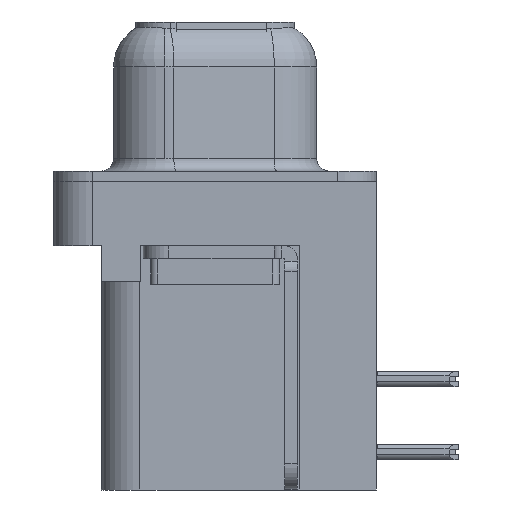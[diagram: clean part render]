
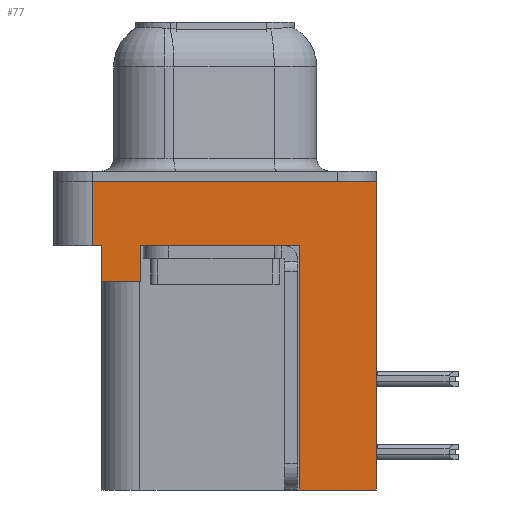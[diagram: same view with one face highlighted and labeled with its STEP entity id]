
A CAD part, left-side view. The second image highlights one B-rep face of the part: STEP entity #77.
In plain terms, the highlighted planar face has unit normal (-1, 0, 0).
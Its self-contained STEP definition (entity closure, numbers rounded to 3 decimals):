
#77 = ADVANCED_FACE ( 'NONE', ( #7146 ), #19064, .T. ) ;
#356 = LINE ( 'NONE', #5273, #6359 ) ;
#1047 = EDGE_CURVE ( 'NONE', #13381, #5297, #17923, .T. ) ;
#1210 = ORIENTED_EDGE ( 'NONE', *, *, #11453, .F. ) ;
#1944 = VECTOR ( 'NONE', #7794, 1000. ) ;
#2473 = DIRECTION ( 'NONE',  ( 0., 0., 1. ) ) ;
#2707 = CARTESIAN_POINT ( 'NONE',  ( -2.935, -6.275, -2.5 ) ) ;
#3245 = ORIENTED_EDGE ( 'NONE', *, *, #8983, .T. ) ;
#3412 = DIRECTION ( 'NONE',  ( 0., -1., 0. ) ) ;
#3508 = VERTEX_POINT ( 'NONE', #21979 ) ;
#3625 = VERTEX_POINT ( 'NONE', #25024 ) ;
#3809 = VERTEX_POINT ( 'NONE', #25561 ) ;
#4331 = CARTESIAN_POINT ( 'NONE',  ( -2.935, 2.895, -2.5 ) ) ;
#4496 = LINE ( 'NONE', #21752, #25029 ) ;
#4504 = CARTESIAN_POINT ( 'NONE',  ( -2.935, -6.275, 0. ) ) ;
#5273 = CARTESIAN_POINT ( 'NONE',  ( -2.935, 4.775, -2.5 ) ) ;
#5297 = VERTEX_POINT ( 'NONE', #22246 ) ;
#5802 = LINE ( 'NONE', #12717, #15302 ) ;
#5838 = VERTEX_POINT ( 'NONE', #4331 ) ;
#6359 = VECTOR ( 'NONE', #2473, 1000. ) ;
#6766 = ORIENTED_EDGE ( 'NONE', *, *, #17180, .F. ) ;
#6968 = CARTESIAN_POINT ( 'NONE',  ( -2.935, -3.295, -2.5 ) ) ;
#6979 = VERTEX_POINT ( 'NONE', #6968 ) ;
#7146 = FACE_OUTER_BOUND ( 'NONE', #14050, .T. ) ;
#7794 = DIRECTION ( 'NONE',  ( 0., 1., 0. ) ) ;
#8135 = CARTESIAN_POINT ( 'NONE',  ( -2.935, -6.275, -12. ) ) ;
#8267 = ORIENTED_EDGE ( 'NONE', *, *, #24013, .F. ) ;
#8983 = EDGE_CURVE ( 'NONE', #5838, #6979, #5802, .T. ) ;
#9283 = CARTESIAN_POINT ( 'NONE',  ( -2.935, 2.895, -3.9 ) ) ;
#9774 = DIRECTION ( 'NONE',  ( 0., 1., 0. ) ) ;
#9793 = ORIENTED_EDGE ( 'NONE', *, *, #12984, .F. ) ;
#10148 = LINE ( 'NONE', #22686, #19032 ) ;
#10779 = VECTOR ( 'NONE', #13722, 1000. ) ;
#11453 = EDGE_CURVE ( 'NONE', #25065, #6979, #21560, .T. ) ;
#11699 = CARTESIAN_POINT ( 'NONE',  ( -2.935, -3.295, -12. ) ) ;
#11892 = VECTOR ( 'NONE', #3412, 1000. ) ;
#11994 = ORIENTED_EDGE ( 'NONE', *, *, #1047, .F. ) ;
#12368 = VECTOR ( 'NONE', #13240, 1000. ) ;
#12553 = DIRECTION ( 'NONE',  ( 0., 0., 1. ) ) ;
#12717 = CARTESIAN_POINT ( 'NONE',  ( -2.935, -6.275, -2.5 ) ) ;
#12846 = ORIENTED_EDGE ( 'NONE', *, *, #20707, .F. ) ;
#12984 = EDGE_CURVE ( 'NONE', #3809, #13381, #356, .T. ) ;
#13240 = DIRECTION ( 'NONE',  ( 0., 0., 1. ) ) ;
#13381 = VERTEX_POINT ( 'NONE', #14259 ) ;
#13383 = VERTEX_POINT ( 'NONE', #8135 ) ;
#13722 = DIRECTION ( 'NONE',  ( 0., 0., 1. ) ) ;
#13874 = EDGE_CURVE ( 'NONE', #3809, #19583, #14739, .T. ) ;
#14050 = EDGE_LOOP ( 'NONE', ( #11994, #9793, #22732, #8267, #12846, #20180, #3245, #1210, #6766, #25427 ) ) ;
#14259 = CARTESIAN_POINT ( 'NONE',  ( -2.935, 4.775, 0. ) ) ;
#14349 = DIRECTION ( 'NONE',  ( 0., -1., 0. ) ) ;
#14739 = LINE ( 'NONE', #17357, #11892 ) ;
#15054 = DIRECTION ( 'NONE',  ( 0., 0., 1. ) ) ;
#15302 = VECTOR ( 'NONE', #14349, 1000. ) ;
#16205 = LINE ( 'NONE', #17935, #1944 ) ;
#16347 = VECTOR ( 'NONE', #24821, 1000. ) ;
#16776 = DIRECTION ( 'NONE',  ( 0., 0., 1. ) ) ;
#16846 = EDGE_CURVE ( 'NONE', #13383, #5297, #10148, .T. ) ;
#16958 = EDGE_CURVE ( 'NONE', #3625, #5838, #24738, .T. ) ;
#17180 = EDGE_CURVE ( 'NONE', #13383, #25065, #4496, .T. ) ;
#17357 = CARTESIAN_POINT ( 'NONE',  ( -2.935, -6.275, -2.5 ) ) ;
#17743 = CARTESIAN_POINT ( 'NONE',  ( -2.935, 4.425, -2.5 ) ) ;
#17745 = CARTESIAN_POINT ( 'NONE',  ( -2.935, -3.295, -12. ) ) ;
#17923 = LINE ( 'NONE', #4504, #16347 ) ;
#17935 = CARTESIAN_POINT ( 'NONE',  ( -2.935, 4.425, -3.9 ) ) ;
#19032 = VECTOR ( 'NONE', #12553, 1000. ) ;
#19064 = PLANE ( 'NONE',  #20747 ) ;
#19583 = VERTEX_POINT ( 'NONE', #17743 ) ;
#20180 = ORIENTED_EDGE ( 'NONE', *, *, #16958, .T. ) ;
#20707 = EDGE_CURVE ( 'NONE', #3625, #3508, #16205, .T. ) ;
#20747 = AXIS2_PLACEMENT_3D ( 'NONE', #2707, #24970, #16776 ) ;
#21560 = LINE ( 'NONE', #11699, #10779 ) ;
#21752 = CARTESIAN_POINT ( 'NONE',  ( -2.935, -3.295, -12. ) ) ;
#21979 = CARTESIAN_POINT ( 'NONE',  ( -2.935, 4.425, -3.9 ) ) ;
#22246 = CARTESIAN_POINT ( 'NONE',  ( -2.935, -6.275, 0. ) ) ;
#22686 = CARTESIAN_POINT ( 'NONE',  ( -2.935, -6.275, -2.5 ) ) ;
#22732 = ORIENTED_EDGE ( 'NONE', *, *, #13874, .T. ) ;
#23964 = VECTOR ( 'NONE', #15054, 1000. ) ;
#24013 = EDGE_CURVE ( 'NONE', #3508, #19583, #26184, .T. ) ;
#24738 = LINE ( 'NONE', #9283, #12368 ) ;
#24821 = DIRECTION ( 'NONE',  ( 0., -1., 0. ) ) ;
#24970 = DIRECTION ( 'NONE',  ( -1., 0., 0. ) ) ;
#25024 = CARTESIAN_POINT ( 'NONE',  ( -2.935, 2.895, -3.9 ) ) ;
#25029 = VECTOR ( 'NONE', #9774, 1000. ) ;
#25065 = VERTEX_POINT ( 'NONE', #17745 ) ;
#25427 = ORIENTED_EDGE ( 'NONE', *, *, #16846, .T. ) ;
#25561 = CARTESIAN_POINT ( 'NONE',  ( -2.935, 4.775, -2.5 ) ) ;
#25566 = CARTESIAN_POINT ( 'NONE',  ( -2.935, 4.425, -3.9 ) ) ;
#26184 = LINE ( 'NONE', #25566, #23964 ) ;
